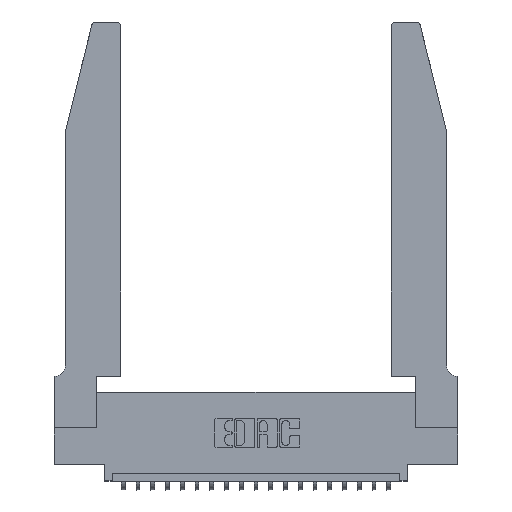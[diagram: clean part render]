
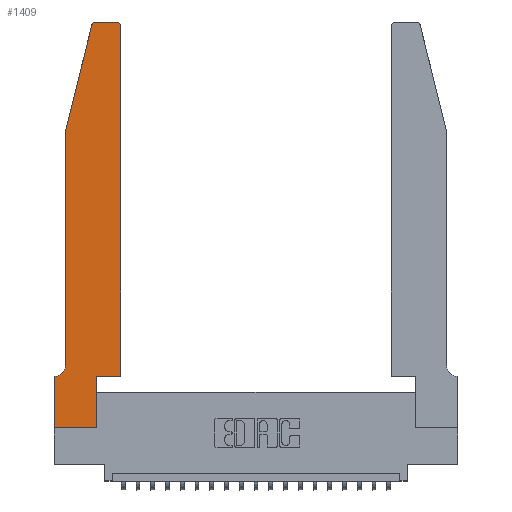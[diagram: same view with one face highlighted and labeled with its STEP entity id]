
A CAD part, top view. The second image highlights one B-rep face of the part: STEP entity #1409.
In plain terms, the highlighted planar face has unit normal (0, 0, 1).
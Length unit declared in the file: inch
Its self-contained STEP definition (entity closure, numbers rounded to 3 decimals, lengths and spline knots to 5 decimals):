
#696 = DIRECTION ( 'NONE',  ( 0., -1., 0. ) ) ;
#794 = CIRCLE ( 'NONE', #20326, 0.03 ) ;
#926 = VERTEX_POINT ( 'NONE', #10385 ) ;
#1409 = ADVANCED_FACE ( 'NONE', ( #14442 ), #22069, .T. ) ;
#1465 = VERTEX_POINT ( 'NONE', #10200 ) ;
#2333 = EDGE_CURVE ( 'NONE', #21260, #4217, #14943, .T. ) ;
#2448 = CARTESIAN_POINT ( 'NONE',  ( 0.0755, 0.35, 0.37 ) ) ;
#2977 = CARTESIAN_POINT ( 'NONE',  ( 0.284, 2.72, 0.37 ) ) ;
#2982 = AXIS2_PLACEMENT_3D ( 'NONE', #14091, #13186, #20225 ) ;
#3003 = CARTESIAN_POINT ( 'NONE',  ( 0.4505, 2.72, 0.37 ) ) ;
#3292 = CARTESIAN_POINT ( 'NONE',  ( 0., 0.35, 0.37 ) ) ;
#3562 = ORIENTED_EDGE ( 'NONE', *, *, #13742, .T. ) ;
#3578 = VECTOR ( 'NONE', #18346, 39.37008 ) ;
#4179 = DIRECTION ( 'NONE',  ( 1., 0., 0. ) ) ;
#4217 = VERTEX_POINT ( 'NONE', #16616 ) ;
#4471 = EDGE_CURVE ( 'NONE', #9764, #12066, #4907, .T. ) ;
#4587 = VERTEX_POINT ( 'NONE', #15568 ) ;
#4667 = VERTEX_POINT ( 'NONE', #19875 ) ;
#4907 = LINE ( 'NONE', #16502, #17887 ) ;
#4935 = CARTESIAN_POINT ( 'NONE',  ( 0.4505, 0.35, 0.37 ) ) ;
#5934 = DIRECTION ( 'NONE',  ( 1., 0., 0. ) ) ;
#6409 = ORIENTED_EDGE ( 'NONE', *, *, #9324, .T. ) ;
#6826 = VECTOR ( 'NONE', #22000, 39.37008 ) ;
#6866 = DIRECTION ( 'NONE',  ( 0., 0., 1. ) ) ;
#7667 = EDGE_CURVE ( 'NONE', #12968, #11011, #21516, .T. ) ;
#7698 = EDGE_CURVE ( 'NONE', #1465, #21305, #19653, .T. ) ;
#7712 = CARTESIAN_POINT ( 'NONE',  ( 0., 0., 0.37 ) ) ;
#7715 = DIRECTION ( 'NONE',  ( -1., 0., 0. ) ) ;
#8603 = CARTESIAN_POINT ( 'NONE',  ( 0., 0.35, 0.37 ) ) ;
#8730 = ORIENTED_EDGE ( 'NONE', *, *, #7667, .T. ) ;
#9095 = ORIENTED_EDGE ( 'NONE', *, *, #9606, .T. ) ;
#9324 = EDGE_CURVE ( 'NONE', #926, #21260, #12847, .T. ) ;
#9434 = CARTESIAN_POINT ( 'NONE',  ( 0.0055, 0.42, 0.37 ) ) ;
#9575 = CARTESIAN_POINT ( 'NONE',  ( 0.4505, 0.35, 0.37 ) ) ;
#9606 = EDGE_CURVE ( 'NONE', #11011, #4587, #18449, .T. ) ;
#9764 = VERTEX_POINT ( 'NONE', #15275 ) ;
#10050 = VECTOR ( 'NONE', #7715, 39.37008 ) ;
#10180 = EDGE_CURVE ( 'NONE', #4217, #12968, #12260, .T. ) ;
#10200 = CARTESIAN_POINT ( 'NONE',  ( 0.0755, 0.42, 0.37 ) ) ;
#10385 = CARTESIAN_POINT ( 'NONE',  ( 0., 0., 0.37 ) ) ;
#11011 = VERTEX_POINT ( 'NONE', #3003 ) ;
#11175 = DIRECTION ( 'NONE',  ( -1., 0., 0. ) ) ;
#11280 = EDGE_CURVE ( 'NONE', #4667, #9764, #794, .T. ) ;
#12066 = VERTEX_POINT ( 'NONE', #16482 ) ;
#12258 = CARTESIAN_POINT ( 'NONE',  ( 0.0055, 0.35, 0.37 ) ) ;
#12260 = LINE ( 'NONE', #19626, #13578 ) ;
#12847 = LINE ( 'NONE', #16257, #16591 ) ;
#12968 = VERTEX_POINT ( 'NONE', #4935 ) ;
#13186 = DIRECTION ( 'NONE',  ( 0., 0., 1. ) ) ;
#13578 = VECTOR ( 'NONE', #4179, 39.37008 ) ;
#13742 = EDGE_CURVE ( 'NONE', #19066, #926, #20397, .T. ) ;
#13869 = DIRECTION ( 'NONE',  ( 1., 0., 0. ) ) ;
#13982 = ORIENTED_EDGE ( 'NONE', *, *, #17469, .T. ) ;
#14091 = CARTESIAN_POINT ( 'NONE',  ( 0.4205, 2.72, 0.37 ) ) ;
#14442 = FACE_OUTER_BOUND ( 'NONE', #17250, .T. ) ;
#14470 = DIRECTION ( 'NONE',  ( 0., -1., 0. ) ) ;
#14715 = LINE ( 'NONE', #19796, #17128 ) ;
#14906 = ORIENTED_EDGE ( 'NONE', *, *, #2333, .T. ) ;
#14943 = LINE ( 'NONE', #21863, #3578 ) ;
#15060 = VECTOR ( 'NONE', #19322, 39.37008 ) ;
#15275 = CARTESIAN_POINT ( 'NONE',  ( 0.25487, 2.72718, 0.37 ) ) ;
#15568 = CARTESIAN_POINT ( 'NONE',  ( 0.4205, 2.75, 0.37 ) ) ;
#15603 = ORIENTED_EDGE ( 'NONE', *, *, #4471, .T. ) ;
#16257 = CARTESIAN_POINT ( 'NONE',  ( 0., 0., 0.37 ) ) ;
#16445 = EDGE_CURVE ( 'NONE', #4587, #4667, #17903, .T. ) ;
#16482 = CARTESIAN_POINT ( 'NONE',  ( 0.0755, 2., 0.37 ) ) ;
#16502 = CARTESIAN_POINT ( 'NONE',  ( 0.0755, 2., 0.37 ) ) ;
#16591 = VECTOR ( 'NONE', #5934, 39.37008 ) ;
#16616 = CARTESIAN_POINT ( 'NONE',  ( 0.2865, 0.35, 0.37 ) ) ;
#16791 = LINE ( 'NONE', #2448, #10050 ) ;
#16894 = CARTESIAN_POINT ( 'NONE',  ( 0.2605, 2.75, 0.37 ) ) ;
#16936 = ORIENTED_EDGE ( 'NONE', *, *, #16445, .T. ) ;
#17128 = VECTOR ( 'NONE', #14470, 39.37008 ) ;
#17250 = EDGE_LOOP ( 'NONE', ( #16936, #21209, #15603, #21452, #20247, #13982, #3562, #6409, #14906, #22339, #8730, #9095 ) ) ;
#17469 = EDGE_CURVE ( 'NONE', #21305, #19066, #16791, .T. ) ;
#17887 = VECTOR ( 'NONE', #18027, 39.37008 ) ;
#17903 = LINE ( 'NONE', #16894, #6826 ) ;
#18005 = DIRECTION ( 'NONE',  ( 0., 0., -1. ) ) ;
#18023 = AXIS2_PLACEMENT_3D ( 'NONE', #9434, #18005, #11175 ) ;
#18027 = DIRECTION ( 'NONE',  ( -0.239, -0.971, 0. ) ) ;
#18346 = DIRECTION ( 'NONE',  ( 0., 1., 0. ) ) ;
#18449 = CIRCLE ( 'NONE', #2982, 0.03 ) ;
#19066 = VERTEX_POINT ( 'NONE', #8603 ) ;
#19194 = AXIS2_PLACEMENT_3D ( 'NONE', #3292, #6866, #22360 ) ;
#19322 = DIRECTION ( 'NONE',  ( 0., 1., 0. ) ) ;
#19626 = CARTESIAN_POINT ( 'NONE',  ( 0.4505, 0.35, 0.37 ) ) ;
#19653 = CIRCLE ( 'NONE', #18023, 0.07 ) ;
#19796 = CARTESIAN_POINT ( 'NONE',  ( 0.0755, 2., 0.37 ) ) ;
#19875 = CARTESIAN_POINT ( 'NONE',  ( 0.284, 2.75, 0.37 ) ) ;
#20225 = DIRECTION ( 'NONE',  ( 1., 0., 0. ) ) ;
#20247 = ORIENTED_EDGE ( 'NONE', *, *, #7698, .T. ) ;
#20319 = DIRECTION ( 'NONE',  ( 0., 0., 1. ) ) ;
#20326 = AXIS2_PLACEMENT_3D ( 'NONE', #2977, #20319, #13869 ) ;
#20397 = LINE ( 'NONE', #7712, #22297 ) ;
#20720 = CARTESIAN_POINT ( 'NONE',  ( 0.2865, 0., 0.37 ) ) ;
#21209 = ORIENTED_EDGE ( 'NONE', *, *, #11280, .T. ) ;
#21260 = VERTEX_POINT ( 'NONE', #20720 ) ;
#21305 = VERTEX_POINT ( 'NONE', #12258 ) ;
#21452 = ORIENTED_EDGE ( 'NONE', *, *, #22158, .T. ) ;
#21516 = LINE ( 'NONE', #9575, #15060 ) ;
#21863 = CARTESIAN_POINT ( 'NONE',  ( 0.2865, 0.35, 0.37 ) ) ;
#22000 = DIRECTION ( 'NONE',  ( -1., 0., 0. ) ) ;
#22069 = PLANE ( 'NONE',  #19194 ) ;
#22158 = EDGE_CURVE ( 'NONE', #12066, #1465, #14715, .T. ) ;
#22297 = VECTOR ( 'NONE', #696, 39.37008 ) ;
#22339 = ORIENTED_EDGE ( 'NONE', *, *, #10180, .T. ) ;
#22360 = DIRECTION ( 'NONE',  ( 1., 0., 0. ) ) ;
